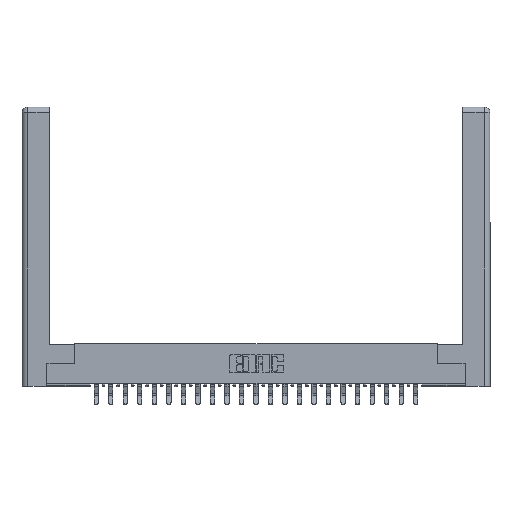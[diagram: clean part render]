
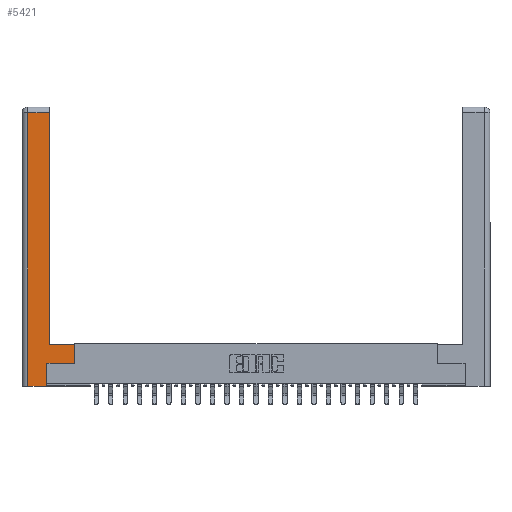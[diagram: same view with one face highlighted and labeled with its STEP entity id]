
A CAD part, top view. The second image highlights one B-rep face of the part: STEP entity #5421.
In plain terms, the highlighted planar face has unit normal (0, 0, 1).
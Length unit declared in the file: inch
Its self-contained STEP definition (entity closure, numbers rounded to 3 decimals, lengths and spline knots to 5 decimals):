
#535 = PLANE ( 'NONE',  #19879 ) ;
#614 = CARTESIAN_POINT ( 'NONE',  ( 0.265, 0.245, 0. ) ) ;
#739 = CARTESIAN_POINT ( 'NONE',  ( 0.565, 0.45, 0. ) ) ;
#2002 = EDGE_LOOP ( 'NONE', ( #26188, #25573, #13413, #17818, #14901, #4971, #5528, #7919 ) ) ;
#2217 = VECTOR ( 'NONE', #27546, 39.37008 ) ;
#2336 = VECTOR ( 'NONE', #15942, 39.37008 ) ;
#2452 = CARTESIAN_POINT ( 'NONE',  ( 0.0615, 2.94, 0. ) ) ;
#2461 = CARTESIAN_POINT ( 'NONE',  ( 0.265, 0.245, 0. ) ) ;
#2820 = VERTEX_POINT ( 'NONE', #10536 ) ;
#4447 = EDGE_CURVE ( 'NONE', #16685, #2820, #26721, .T. ) ;
#4971 = ORIENTED_EDGE ( 'NONE', *, *, #10452, .T. ) ;
#5214 = CARTESIAN_POINT ( 'NONE',  ( 0., 0., 0. ) ) ;
#5421 = ADVANCED_FACE ( 'NONE', ( #25946 ), #535, .F. ) ;
#5528 = ORIENTED_EDGE ( 'NONE', *, *, #18052, .T. ) ;
#5816 = DIRECTION ( 'NONE',  ( 1., 0., 0. ) ) ;
#6248 = VECTOR ( 'NONE', #8173, 39.37008 ) ;
#6595 = VERTEX_POINT ( 'NONE', #11444 ) ;
#6751 = DIRECTION ( 'NONE',  ( 0., 1., 0. ) ) ;
#6917 = LINE ( 'NONE', #25122, #2217 ) ;
#7919 = ORIENTED_EDGE ( 'NONE', *, *, #21254, .T. ) ;
#8173 = DIRECTION ( 'NONE',  ( -1., 0., 0. ) ) ;
#9413 = EDGE_CURVE ( 'NONE', #19187, #6595, #10092, .T. ) ;
#9501 = LINE ( 'NONE', #614, #18951 ) ;
#10092 = LINE ( 'NONE', #22164, #21318 ) ;
#10143 = DIRECTION ( 'NONE',  ( 0., 1., 0. ) ) ;
#10452 = EDGE_CURVE ( 'NONE', #18848, #27720, #28080, .T. ) ;
#10536 = CARTESIAN_POINT ( 'NONE',  ( 0.295, 2.94, 0. ) ) ;
#10782 = CARTESIAN_POINT ( 'NONE',  ( 0.565, 0.245, 0. ) ) ;
#10908 = EDGE_CURVE ( 'NONE', #26208, #18848, #9501, .T. ) ;
#11168 = CARTESIAN_POINT ( 'NONE',  ( 0.565, 0.45, 0. ) ) ;
#11340 = LINE ( 'NONE', #22193, #6248 ) ;
#11444 = CARTESIAN_POINT ( 'NONE',  ( 0.0615, 0., 0. ) ) ;
#12515 = DIRECTION ( 'NONE',  ( -1., 0., 0. ) ) ;
#13413 = ORIENTED_EDGE ( 'NONE', *, *, #9413, .T. ) ;
#14767 = DIRECTION ( 'NONE',  ( 0., 0., -1. ) ) ;
#14901 = ORIENTED_EDGE ( 'NONE', *, *, #10908, .T. ) ;
#15942 = DIRECTION ( 'NONE',  ( 0., 1., 0. ) ) ;
#16685 = VERTEX_POINT ( 'NONE', #21129 ) ;
#17818 = ORIENTED_EDGE ( 'NONE', *, *, #25948, .T. ) ;
#18052 = EDGE_CURVE ( 'NONE', #27720, #26791, #22723, .T. ) ;
#18848 = VERTEX_POINT ( 'NONE', #2461 ) ;
#18951 = VECTOR ( 'NONE', #10143, 39.37008 ) ;
#19187 = VERTEX_POINT ( 'NONE', #2452 ) ;
#19879 = AXIS2_PLACEMENT_3D ( 'NONE', #5214, #14767, #12515 ) ;
#20140 = DIRECTION ( 'NONE',  ( 0., -1., 0. ) ) ;
#20568 = VECTOR ( 'NONE', #6751, 39.37008 ) ;
#20816 = VECTOR ( 'NONE', #5816, 39.37008 ) ;
#21129 = CARTESIAN_POINT ( 'NONE',  ( 0.295, 0.45, 0. ) ) ;
#21254 = EDGE_CURVE ( 'NONE', #26791, #16685, #11340, .T. ) ;
#21318 = VECTOR ( 'NONE', #20140, 39.37008 ) ;
#21342 = CARTESIAN_POINT ( 'NONE',  ( 0.565, 0.245, 0. ) ) ;
#22164 = CARTESIAN_POINT ( 'NONE',  ( 0.0615, 0., 0. ) ) ;
#22193 = CARTESIAN_POINT ( 'NONE',  ( 0.295, 0.45, 0. ) ) ;
#22723 = LINE ( 'NONE', #11168, #2336 ) ;
#23553 = CARTESIAN_POINT ( 'NONE',  ( 0.265, 0., 0. ) ) ;
#24867 = CARTESIAN_POINT ( 'NONE',  ( 0.0615, 2.94, 0. ) ) ;
#25122 = CARTESIAN_POINT ( 'NONE',  ( 0.265, 0., 0. ) ) ;
#25573 = ORIENTED_EDGE ( 'NONE', *, *, #27427, .T. ) ;
#25946 = FACE_OUTER_BOUND ( 'NONE', #2002, .T. ) ;
#25948 = EDGE_CURVE ( 'NONE', #6595, #26208, #6917, .T. ) ;
#26188 = ORIENTED_EDGE ( 'NONE', *, *, #4447, .T. ) ;
#26208 = VERTEX_POINT ( 'NONE', #23553 ) ;
#26721 = LINE ( 'NONE', #27697, #20568 ) ;
#26791 = VERTEX_POINT ( 'NONE', #739 ) ;
#26837 = LINE ( 'NONE', #24867, #27585 ) ;
#27427 = EDGE_CURVE ( 'NONE', #2820, #19187, #26837, .T. ) ;
#27546 = DIRECTION ( 'NONE',  ( 1., 0., 0. ) ) ;
#27585 = VECTOR ( 'NONE', #29218, 39.37008 ) ;
#27697 = CARTESIAN_POINT ( 'NONE',  ( 0.295, 3., 0. ) ) ;
#27720 = VERTEX_POINT ( 'NONE', #21342 ) ;
#28080 = LINE ( 'NONE', #10782, #20816 ) ;
#29218 = DIRECTION ( 'NONE',  ( -1., 0., 0. ) ) ;
